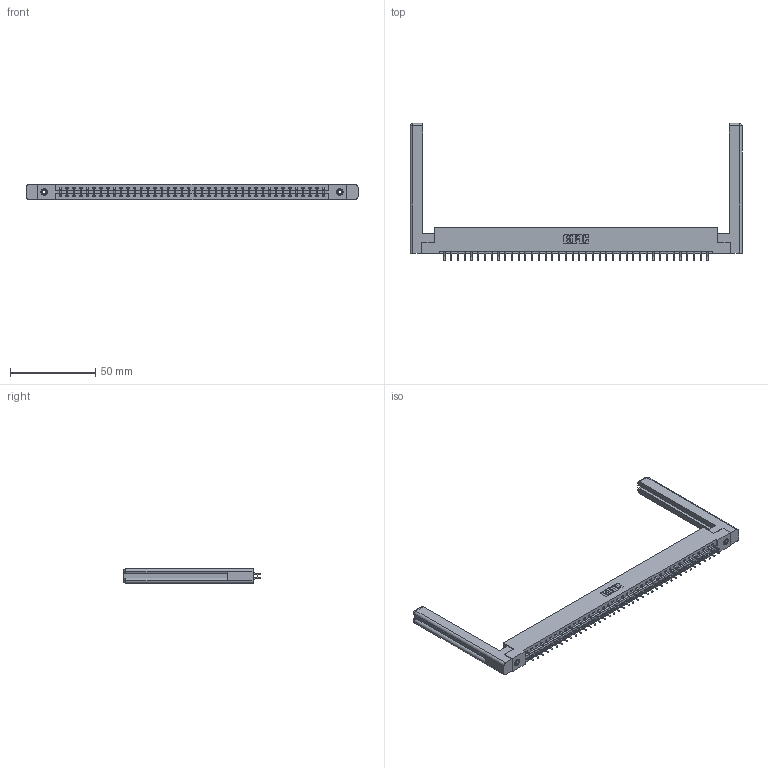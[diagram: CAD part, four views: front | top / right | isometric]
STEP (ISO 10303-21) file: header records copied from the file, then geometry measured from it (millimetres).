
FILE_DESCRIPTION (( 'STEP AP203' ), '1' );
FILE_NAME ('337-080-556-258.STEP', '2019-10-10T12:29:43', ( '' ), ( '' ), 'SwSTEP 2.0', 'SolidWorks 2016', '' );
FILE_SCHEMA (( 'CONFIG_CONTROL_DESIGN' ));
Length unit declared in the file: inch
Products named in the file (5): 337 Part_Flush Mounting Lugs - 0.156 Dia-TI; 307-220-058; 337-080-556-258; 345-292-001_556 Tail; 345-250-001_345-250-001-102
Assembly tree (85 placements, depth 2):
  337-080-556-258
    337 Part_Flush Mounting Lugs - 0.156 Dia-TI
    345-292-001_556 Tail  x80
    345-250-001_345-250-001-102  x2
    307-220-058  x2
Bounding box: 195.12 x 80.66 x 9.4 mm (x, y, z)
Volume: 27676.1 mm3; surface area: 28156.4 mm2
Topology: 85 solids, 85 shells, 5056 faces, 14985 edges, 9870 vertices
Faces by surface type: plane 3514, cylinder 1518, cone 12, torus 12
Entity records: 34126 total; most frequent: CARTESIAN_POINT 5773, ORIENTED_EDGE 5636, DIRECTION 4918, EDGE_CURVE 2818, LINE 2634, VECTOR 2634, VERTEX_POINT 1870, AXIS2_PLACEMENT_3D 1142
